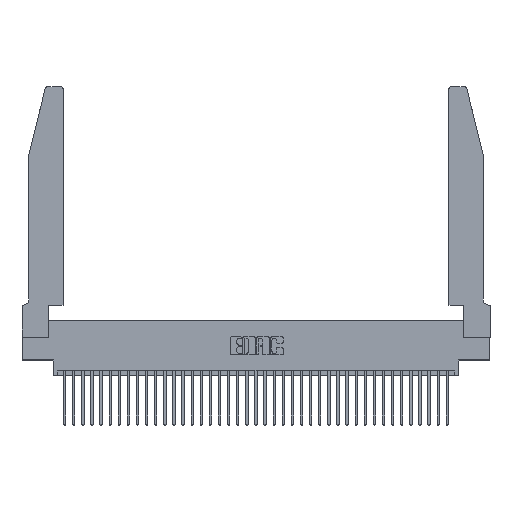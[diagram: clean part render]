
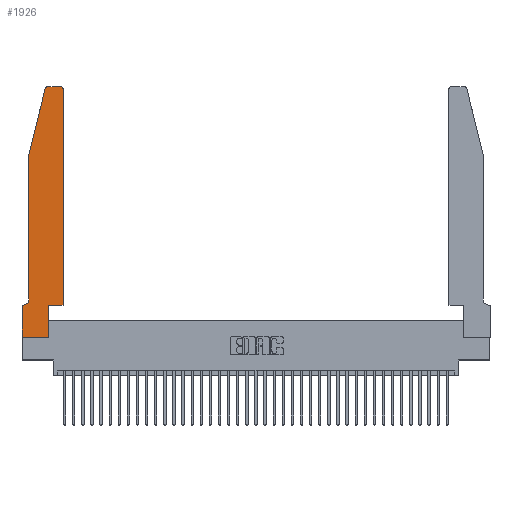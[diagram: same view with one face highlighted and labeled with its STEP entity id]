
A CAD part, top view. The second image highlights one B-rep face of the part: STEP entity #1926.
In plain terms, the highlighted planar face has unit normal (0, 0, 1).
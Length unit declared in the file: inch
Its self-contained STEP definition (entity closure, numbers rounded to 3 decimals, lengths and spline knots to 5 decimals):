
#372 = CARTESIAN_POINT ( 'NONE',  ( 0.4505, 0.35, 0.37 ) ) ;
#650 = CARTESIAN_POINT ( 'NONE',  ( 0.284, 2.72, 0.37 ) ) ;
#1337 = VERTEX_POINT ( 'NONE', #2662 ) ;
#1358 = CIRCLE ( 'NONE', #12596, 0.03 ) ;
#1472 = ORIENTED_EDGE ( 'NONE', *, *, #15004, .T. ) ;
#1608 = CARTESIAN_POINT ( 'NONE',  ( 0.0055, 0.42, 0.37 ) ) ;
#1895 = VECTOR ( 'NONE', #1961, 39.37008 ) ;
#1926 = ADVANCED_FACE ( 'NONE', ( #16348 ), #21200, .T. ) ;
#1961 = DIRECTION ( 'NONE',  ( -1., 0., 0. ) ) ;
#2662 = CARTESIAN_POINT ( 'NONE',  ( 0.2865, 0., 0.37 ) ) ;
#2808 = DIRECTION ( 'NONE',  ( 0., 1., 0. ) ) ;
#2906 = DIRECTION ( 'NONE',  ( 1., 0., 0. ) ) ;
#3347 = CARTESIAN_POINT ( 'NONE',  ( 0.4505, 0.35, 0.37 ) ) ;
#3352 = CARTESIAN_POINT ( 'NONE',  ( 0., 0.35, 0.37 ) ) ;
#4737 = ORIENTED_EDGE ( 'NONE', *, *, #20902, .T. ) ;
#6301 = CARTESIAN_POINT ( 'NONE',  ( 0.0755, 2., 0.37 ) ) ;
#6325 = ORIENTED_EDGE ( 'NONE', *, *, #36650, .T. ) ;
#6451 = DIRECTION ( 'NONE',  ( 1., 0., 0. ) ) ;
#6687 = ORIENTED_EDGE ( 'NONE', *, *, #22711, .T. ) ;
#6953 = CARTESIAN_POINT ( 'NONE',  ( 0.0755, 0.35, 0.37 ) ) ;
#7014 = VECTOR ( 'NONE', #2808, 39.37008 ) ;
#7533 = EDGE_CURVE ( 'NONE', #38202, #15180, #28550, .T. ) ;
#7781 = LINE ( 'NONE', #29307, #30531 ) ;
#8122 = CARTESIAN_POINT ( 'NONE',  ( 0.0755, 0.42, 0.37 ) ) ;
#8938 = CARTESIAN_POINT ( 'NONE',  ( 0.4505, 0.35, 0.37 ) ) ;
#9191 = DIRECTION ( 'NONE',  ( 0., 1., 0. ) ) ;
#9348 = VERTEX_POINT ( 'NONE', #29913 ) ;
#10159 = LINE ( 'NONE', #10977, #25444 ) ;
#10176 = ORIENTED_EDGE ( 'NONE', *, *, #14144, .T. ) ;
#10264 = EDGE_CURVE ( 'NONE', #22497, #32980, #24119, .T. ) ;
#10775 = VERTEX_POINT ( 'NONE', #27742 ) ;
#10977 = CARTESIAN_POINT ( 'NONE',  ( 0.0755, 2., 0.37 ) ) ;
#12316 = EDGE_CURVE ( 'NONE', #32980, #1337, #32815, .T. ) ;
#12574 = VECTOR ( 'NONE', #18184, 39.37008 ) ;
#12596 = AXIS2_PLACEMENT_3D ( 'NONE', #31689, #31818, #16971 ) ;
#12932 = CARTESIAN_POINT ( 'NONE',  ( 0.4205, 2.75, 0.37 ) ) ;
#13151 = CARTESIAN_POINT ( 'NONE',  ( 0., 0., 0.37 ) ) ;
#13607 = ORIENTED_EDGE ( 'NONE', *, *, #12316, .T. ) ;
#14144 = EDGE_CURVE ( 'NONE', #15180, #32224, #1358, .T. ) ;
#14891 = DIRECTION ( 'NONE',  ( -0.239, -0.971, 0. ) ) ;
#14897 = LINE ( 'NONE', #37925, #7014 ) ;
#15004 = EDGE_CURVE ( 'NONE', #29836, #36643, #10159, .T. ) ;
#15180 = VERTEX_POINT ( 'NONE', #25132 ) ;
#16104 = AXIS2_PLACEMENT_3D ( 'NONE', #650, #34328, #25227 ) ;
#16181 = EDGE_LOOP ( 'NONE', ( #6687, #24367, #19184, #1472, #18305, #31958, #27339, #13607, #4737, #6325, #34372, #10176 ) ) ;
#16348 = FACE_OUTER_BOUND ( 'NONE', #16181, .T. ) ;
#16541 = EDGE_CURVE ( 'NONE', #9348, #26163, #16968, .T. ) ;
#16968 = CIRCLE ( 'NONE', #16104, 0.03 ) ;
#16971 = DIRECTION ( 'NONE',  ( 1., 0., 0. ) ) ;
#18184 = DIRECTION ( 'NONE',  ( 1., 0., 0. ) ) ;
#18305 = ORIENTED_EDGE ( 'NONE', *, *, #28559, .T. ) ;
#18496 = CIRCLE ( 'NONE', #22762, 0.07 ) ;
#19184 = ORIENTED_EDGE ( 'NONE', *, *, #31983, .T. ) ;
#20582 = CARTESIAN_POINT ( 'NONE',  ( 0.0755, 2., 0.37 ) ) ;
#20675 = CARTESIAN_POINT ( 'NONE',  ( 0., 0., 0.37 ) ) ;
#20902 = EDGE_CURVE ( 'NONE', #1337, #27244, #14897, .T. ) ;
#21200 = PLANE ( 'NONE',  #30054 ) ;
#22266 = DIRECTION ( 'NONE',  ( 0., -1., 0. ) ) ;
#22497 = VERTEX_POINT ( 'NONE', #3352 ) ;
#22711 = EDGE_CURVE ( 'NONE', #32224, #9348, #7781, .T. ) ;
#22762 = AXIS2_PLACEMENT_3D ( 'NONE', #1608, #28246, #36969 ) ;
#23423 = VECTOR ( 'NONE', #9191, 39.37008 ) ;
#24119 = LINE ( 'NONE', #25268, #26477 ) ;
#24226 = DIRECTION ( 'NONE',  ( 0., 0., 1. ) ) ;
#24293 = LINE ( 'NONE', #20582, #27538 ) ;
#24367 = ORIENTED_EDGE ( 'NONE', *, *, #16541, .T. ) ;
#25132 = CARTESIAN_POINT ( 'NONE',  ( 0.4505, 2.72, 0.37 ) ) ;
#25227 = DIRECTION ( 'NONE',  ( 1., 0., 0. ) ) ;
#25268 = CARTESIAN_POINT ( 'NONE',  ( 0., 0., 0.37 ) ) ;
#25444 = VECTOR ( 'NONE', #26919, 39.37008 ) ;
#26163 = VERTEX_POINT ( 'NONE', #28844 ) ;
#26460 = DIRECTION ( 'NONE',  ( -1., 0., 0. ) ) ;
#26477 = VECTOR ( 'NONE', #22266, 39.37008 ) ;
#26764 = VECTOR ( 'NONE', #2906, 39.37008 ) ;
#26919 = DIRECTION ( 'NONE',  ( 0., -1., 0. ) ) ;
#27221 = EDGE_CURVE ( 'NONE', #10775, #22497, #27929, .T. ) ;
#27244 = VERTEX_POINT ( 'NONE', #37843 ) ;
#27339 = ORIENTED_EDGE ( 'NONE', *, *, #10264, .T. ) ;
#27538 = VECTOR ( 'NONE', #14891, 39.37008 ) ;
#27742 = CARTESIAN_POINT ( 'NONE',  ( 0.0055, 0.35, 0.37 ) ) ;
#27929 = LINE ( 'NONE', #6953, #1895 ) ;
#28246 = DIRECTION ( 'NONE',  ( 0., 0., -1. ) ) ;
#28355 = LINE ( 'NONE', #372, #12574 ) ;
#28550 = LINE ( 'NONE', #8938, #23423 ) ;
#28559 = EDGE_CURVE ( 'NONE', #36643, #10775, #18496, .T. ) ;
#28844 = CARTESIAN_POINT ( 'NONE',  ( 0.25487, 2.72718, 0.37 ) ) ;
#29307 = CARTESIAN_POINT ( 'NONE',  ( 0.2605, 2.75, 0.37 ) ) ;
#29836 = VERTEX_POINT ( 'NONE', #6301 ) ;
#29913 = CARTESIAN_POINT ( 'NONE',  ( 0.284, 2.75, 0.37 ) ) ;
#30054 = AXIS2_PLACEMENT_3D ( 'NONE', #33210, #24226, #6451 ) ;
#30531 = VECTOR ( 'NONE', #26460, 39.37008 ) ;
#31689 = CARTESIAN_POINT ( 'NONE',  ( 0.4205, 2.72, 0.37 ) ) ;
#31818 = DIRECTION ( 'NONE',  ( 0., 0., 1. ) ) ;
#31958 = ORIENTED_EDGE ( 'NONE', *, *, #27221, .T. ) ;
#31983 = EDGE_CURVE ( 'NONE', #26163, #29836, #24293, .T. ) ;
#32224 = VERTEX_POINT ( 'NONE', #12932 ) ;
#32815 = LINE ( 'NONE', #20675, #26764 ) ;
#32980 = VERTEX_POINT ( 'NONE', #13151 ) ;
#33210 = CARTESIAN_POINT ( 'NONE',  ( 0., 0.35, 0.37 ) ) ;
#34328 = DIRECTION ( 'NONE',  ( 0., 0., 1. ) ) ;
#34372 = ORIENTED_EDGE ( 'NONE', *, *, #7533, .T. ) ;
#36643 = VERTEX_POINT ( 'NONE', #8122 ) ;
#36650 = EDGE_CURVE ( 'NONE', #27244, #38202, #28355, .T. ) ;
#36969 = DIRECTION ( 'NONE',  ( -1., 0., 0. ) ) ;
#37843 = CARTESIAN_POINT ( 'NONE',  ( 0.2865, 0.35, 0.37 ) ) ;
#37925 = CARTESIAN_POINT ( 'NONE',  ( 0.2865, 0.35, 0.37 ) ) ;
#38202 = VERTEX_POINT ( 'NONE', #3347 ) ;
